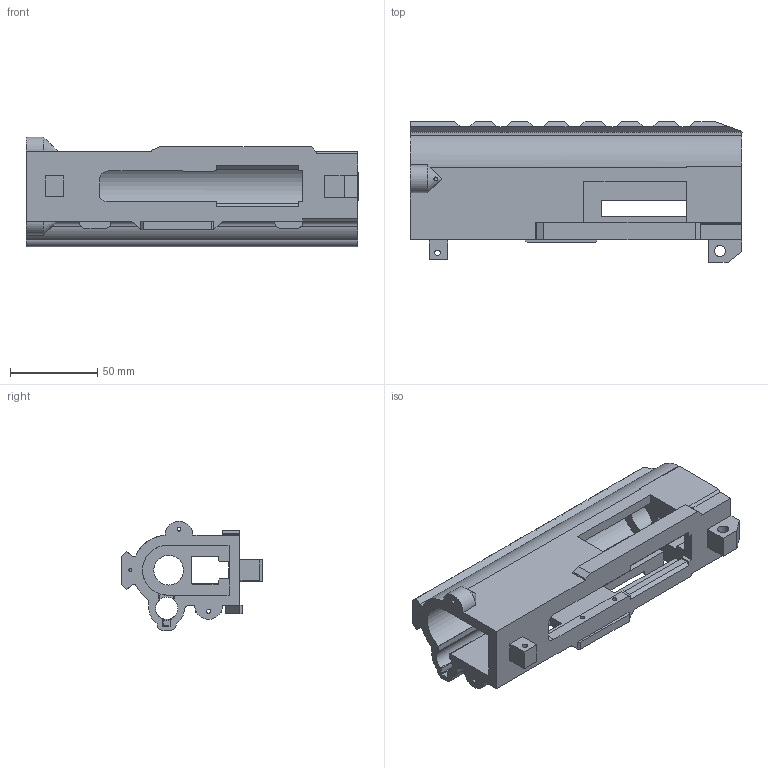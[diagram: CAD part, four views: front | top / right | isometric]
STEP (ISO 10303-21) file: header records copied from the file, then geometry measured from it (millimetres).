
FILE_DESCRIPTION (( 'STEP AP203' ), '1' );
FILE_NAME ('WTF-9_upper_receiver.STEP', '2020-05-09T09:17:03', ( '' ), ( '' ), 'SwSTEP 2.0', 'SolidWorks 2016', '' );
FILE_SCHEMA (( 'CONFIG_CONTROL_DESIGN' ));
Length unit declared in the file: millimetre
Products named in the file (2): WTF-9_upper_receiver; WTF9 V1 FINAL_9
Assembly tree (1 placements, depth 2):
  WTF-9_upper_receiver
    WTF9 V1 FINAL_9
Bounding box: 190.38 x 80.5 x 62.82 mm (x, y, z)
Volume: 229551.4 mm3; surface area: 81524 mm2
Topology: 1 solids, 1 shells, 281 faces, 788 edges, 507 vertices
Faces by surface type: plane 214, cylinder 50, cone 8, torus 5, sphere 2, bspline 2
Full cylindrical faces by diameter (mm): 1.7 x1, 2.2 x1, 2.4 x5, 2.6 x2, 3.175 x1, 6.375 x1, 12.8 x1, 17 x1
Entity records: 9222 total; most frequent: CARTESIAN_POINT 1804, ORIENTED_EDGE 1530, DIRECTION 1419, EDGE_CURVE 765, VECTOR 637, LINE 637, VERTEX_POINT 504, AXIS2_PLACEMENT_3D 391
